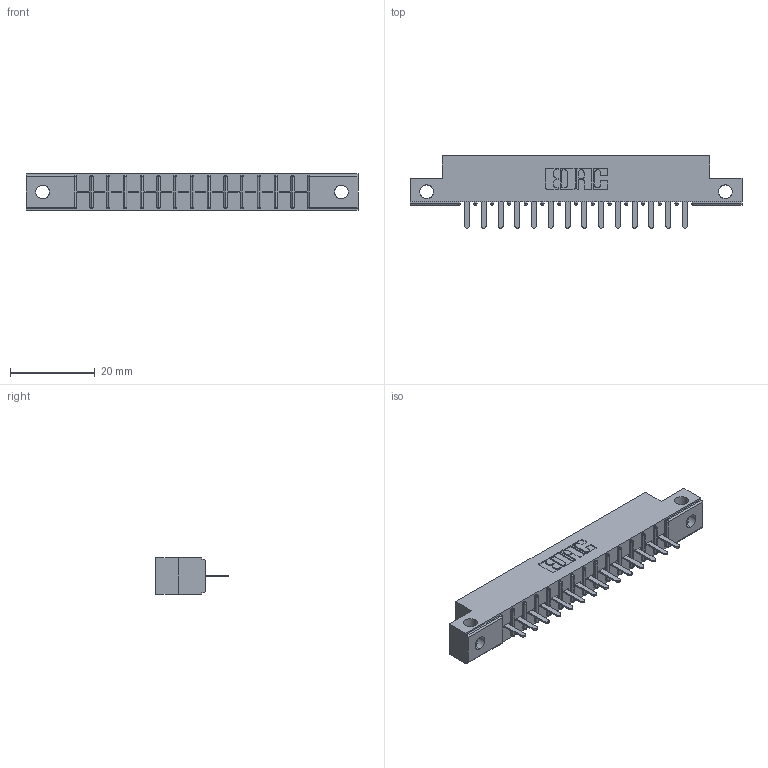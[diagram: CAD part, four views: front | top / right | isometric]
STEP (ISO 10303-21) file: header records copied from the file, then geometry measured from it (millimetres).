
FILE_DESCRIPTION (( 'STEP AP203' ), '1' );
FILE_NAME ('306-014-420-112.STEP', '2020-09-21T17:56:05', ( '' ), ( '' ), 'SwSTEP 2.0', 'SolidWorks 2020', '' );
FILE_SCHEMA (( 'CONFIG_CONTROL_DESIGN' ));
Length unit declared in the file: inch
Products named in the file (3): 306-014-420-112; 306 Part_.128 Dia; 306-290-001_120
Assembly tree (15 placements, depth 2):
  306-014-420-112
    306 Part_.128 Dia
    306-290-001_120  x14
Bounding box: 78.49 x 17.12 x 8.71 mm (x, y, z)
Volume: 5195.1 mm3; surface area: 7384.7 mm2
Topology: 15 solids, 15 shells, 1108 faces, 3110 edges, 1992 vertices
Faces by surface type: plane 726, cylinder 326, sphere 56
Entity records: 17045 total; most frequent: CARTESIAN_POINT 2905, ORIENTED_EDGE 2832, DIRECTION 2806, EDGE_CURVE 1416, LINE 1076, VECTOR 1076, VERTEX_POINT 900, AXIS2_PLACEMENT_3D 865
